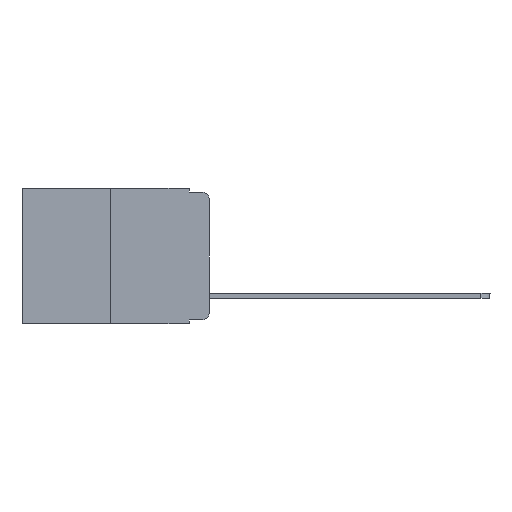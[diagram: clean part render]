
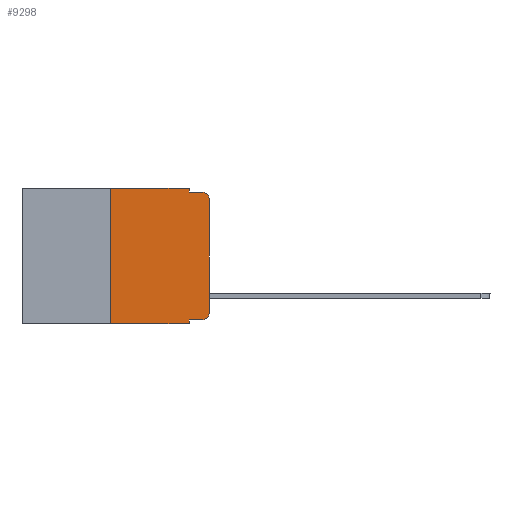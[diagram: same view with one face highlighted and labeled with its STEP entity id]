
A CAD part, left-side view. The second image highlights one B-rep face of the part: STEP entity #9298.
In plain terms, the highlighted planar face has unit normal (-1, 0, 0).
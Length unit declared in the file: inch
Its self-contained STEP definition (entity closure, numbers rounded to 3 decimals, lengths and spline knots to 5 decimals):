
#19 = DIRECTION ( 'NONE',  ( 0., 0., 1. ) ) ;
#85 = EDGE_CURVE ( 'NONE', #2534, #3649, #923, .T. ) ;
#194 = AXIS2_PLACEMENT_3D ( 'NONE', #8202, #9012, #8163 ) ;
#339 = DIRECTION ( 'NONE',  ( 0., 0., -1. ) ) ;
#377 = LINE ( 'NONE', #941, #4491 ) ;
#389 = DIRECTION ( 'NONE',  ( 0., -1., 0. ) ) ;
#450 = ORIENTED_EDGE ( 'NONE', *, *, #10396, .T. ) ;
#547 = VECTOR ( 'NONE', #9463, 39.37008 ) ;
#629 = CARTESIAN_POINT ( 'NONE',  ( 0., 0.051, -0.01 ) ) ;
#844 = ORIENTED_EDGE ( 'NONE', *, *, #10061, .F. ) ;
#851 = AXIS2_PLACEMENT_3D ( 'NONE', #7931, #8037, #339 ) ;
#884 = VERTEX_POINT ( 'NONE', #9024 ) ;
#923 = CIRCLE ( 'NONE', #851, 0.02 ) ;
#941 = CARTESIAN_POINT ( 'NONE',  ( 0., 0.473, -0.343 ) ) ;
#1076 = EDGE_CURVE ( 'NONE', #1634, #9379, #1764, .T. ) ;
#1117 = DIRECTION ( 'NONE',  ( 0., 0., -1. ) ) ;
#1148 = CARTESIAN_POINT ( 'NONE',  ( 0., 0.051, -0.333 ) ) ;
#1204 = VERTEX_POINT ( 'NONE', #6817 ) ;
#1380 = CARTESIAN_POINT ( 'NONE',  ( 0., 0.25, 0. ) ) ;
#1634 = VERTEX_POINT ( 'NONE', #5688 ) ;
#1764 = LINE ( 'NONE', #7430, #6919 ) ;
#1815 = DIRECTION ( 'NONE',  ( 0., -1., 0. ) ) ;
#1855 = DIRECTION ( 'NONE',  ( 0., -1., 0. ) ) ;
#1942 = CARTESIAN_POINT ( 'NONE',  ( 0., 0.051, 0. ) ) ;
#2062 = CIRCLE ( 'NONE', #6398, 0.02 ) ;
#2230 = FACE_OUTER_BOUND ( 'NONE', #4429, .T. ) ;
#2534 = VERTEX_POINT ( 'NONE', #6786 ) ;
#2926 = CARTESIAN_POINT ( 'NONE',  ( 0., 0.02, -0.01 ) ) ;
#3051 = EDGE_CURVE ( 'NONE', #1634, #10391, #377, .T. ) ;
#3321 = CARTESIAN_POINT ( 'NONE',  ( 0., 0.051, -0.343 ) ) ;
#3371 = LINE ( 'NONE', #4258, #10944 ) ;
#3412 = VECTOR ( 'NONE', #6795, 39.37008 ) ;
#3431 = EDGE_CURVE ( 'NONE', #1204, #2534, #7608, .T. ) ;
#3544 = CARTESIAN_POINT ( 'NONE',  ( 0., 0.473, 0. ) ) ;
#3649 = VERTEX_POINT ( 'NONE', #5376 ) ;
#4019 = VECTOR ( 'NONE', #1855, 39.37008 ) ;
#4258 = CARTESIAN_POINT ( 'NONE',  ( 0., 0., 0. ) ) ;
#4429 = EDGE_LOOP ( 'NONE', ( #8821, #450, #844, #6860, #6991, #6146, #9240, #8469, #5755, #8488 ) ) ;
#4491 = VECTOR ( 'NONE', #1815, 39.37008 ) ;
#4602 = VERTEX_POINT ( 'NONE', #2926 ) ;
#4909 = EDGE_CURVE ( 'NONE', #3649, #8473, #3371, .T. ) ;
#5023 = DIRECTION ( 'NONE',  ( -1., 0., 0. ) ) ;
#5180 = CARTESIAN_POINT ( 'NONE',  ( 0., 0., -0.03 ) ) ;
#5188 = EDGE_CURVE ( 'NONE', #9379, #884, #7882, .T. ) ;
#5376 = CARTESIAN_POINT ( 'NONE',  ( 0., 0., -0.313 ) ) ;
#5461 = CARTESIAN_POINT ( 'NONE',  ( 0., 0.051, -0.01 ) ) ;
#5519 = LINE ( 'NONE', #5461, #9146 ) ;
#5688 = CARTESIAN_POINT ( 'NONE',  ( 0., 0.25, -0.343 ) ) ;
#5755 = ORIENTED_EDGE ( 'NONE', *, *, #3431, .T. ) ;
#6093 = VERTEX_POINT ( 'NONE', #629 ) ;
#6146 = ORIENTED_EDGE ( 'NONE', *, *, #1076, .F. ) ;
#6398 = AXIS2_PLACEMENT_3D ( 'NONE', #9283, #5023, #10984 ) ;
#6499 = LINE ( 'NONE', #1942, #6758 ) ;
#6758 = VECTOR ( 'NONE', #1117, 39.37008 ) ;
#6786 = CARTESIAN_POINT ( 'NONE',  ( 0., 0.02, -0.333 ) ) ;
#6795 = DIRECTION ( 'NONE',  ( 0., 0., -1. ) ) ;
#6817 = CARTESIAN_POINT ( 'NONE',  ( 0., 0.051, -0.333 ) ) ;
#6860 = ORIENTED_EDGE ( 'NONE', *, *, #10986, .F. ) ;
#6919 = VECTOR ( 'NONE', #7461, 39.37008 ) ;
#6991 = ORIENTED_EDGE ( 'NONE', *, *, #5188, .F. ) ;
#7430 = CARTESIAN_POINT ( 'NONE',  ( 0., 0.25, 0. ) ) ;
#7461 = DIRECTION ( 'NONE',  ( 0., 0., 1. ) ) ;
#7608 = LINE ( 'NONE', #1148, #4019 ) ;
#7795 = LINE ( 'NONE', #10007, #3412 ) ;
#7882 = LINE ( 'NONE', #3544, #547 ) ;
#7931 = CARTESIAN_POINT ( 'NONE',  ( 0., 0.02, -0.313 ) ) ;
#8037 = DIRECTION ( 'NONE',  ( -1., 0., 0. ) ) ;
#8163 = DIRECTION ( 'NONE',  ( 0., 0., -1. ) ) ;
#8202 = CARTESIAN_POINT ( 'NONE',  ( 0., 0.473, 0. ) ) ;
#8469 = ORIENTED_EDGE ( 'NONE', *, *, #9213, .F. ) ;
#8473 = VERTEX_POINT ( 'NONE', #5180 ) ;
#8488 = ORIENTED_EDGE ( 'NONE', *, *, #85, .T. ) ;
#8821 = ORIENTED_EDGE ( 'NONE', *, *, #4909, .T. ) ;
#9012 = DIRECTION ( 'NONE',  ( 1., 0., 0. ) ) ;
#9024 = CARTESIAN_POINT ( 'NONE',  ( 0., 0.051, 0. ) ) ;
#9146 = VECTOR ( 'NONE', #389, 39.37008 ) ;
#9213 = EDGE_CURVE ( 'NONE', #1204, #10391, #6499, .T. ) ;
#9240 = ORIENTED_EDGE ( 'NONE', *, *, #3051, .T. ) ;
#9283 = CARTESIAN_POINT ( 'NONE',  ( 0., 0.02, -0.03 ) ) ;
#9298 = ADVANCED_FACE ( 'NONE', ( #2230 ), #9624, .F. ) ;
#9379 = VERTEX_POINT ( 'NONE', #1380 ) ;
#9463 = DIRECTION ( 'NONE',  ( 0., -1., 0. ) ) ;
#9624 = PLANE ( 'NONE',  #194 ) ;
#10007 = CARTESIAN_POINT ( 'NONE',  ( 0., 0.051, 0. ) ) ;
#10061 = EDGE_CURVE ( 'NONE', #6093, #4602, #5519, .T. ) ;
#10391 = VERTEX_POINT ( 'NONE', #3321 ) ;
#10396 = EDGE_CURVE ( 'NONE', #8473, #4602, #2062, .T. ) ;
#10944 = VECTOR ( 'NONE', #19, 39.37008 ) ;
#10984 = DIRECTION ( 'NONE',  ( 0., 0., -1. ) ) ;
#10986 = EDGE_CURVE ( 'NONE', #884, #6093, #7795, .T. ) ;
